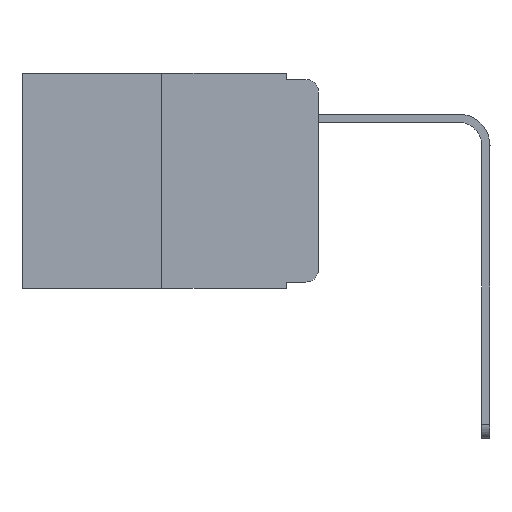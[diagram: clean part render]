
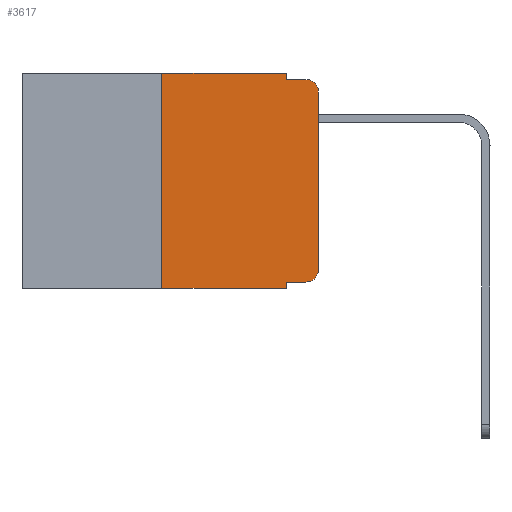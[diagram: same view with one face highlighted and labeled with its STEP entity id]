
A CAD part, left-side view. The second image highlights one B-rep face of the part: STEP entity #3617.
In plain terms, the highlighted planar face has unit normal (-1, 0, 0).
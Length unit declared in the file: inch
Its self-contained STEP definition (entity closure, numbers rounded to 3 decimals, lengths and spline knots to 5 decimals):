
#170 = CARTESIAN_POINT ( 'NONE',  ( 0., 0.02, -0.313 ) ) ;
#175 = VECTOR ( 'NONE', #9931, 39.37008 ) ;
#216 = CARTESIAN_POINT ( 'NONE',  ( 0., 0.02, -0.333 ) ) ;
#273 = LINE ( 'NONE', #3602, #7052 ) ;
#281 = DIRECTION ( 'NONE',  ( 0., 0., -1. ) ) ;
#311 = VERTEX_POINT ( 'NONE', #536 ) ;
#536 = CARTESIAN_POINT ( 'NONE',  ( 0., 0.051, -0.333 ) ) ;
#756 = CARTESIAN_POINT ( 'NONE',  ( 0., 0.051, -0.01 ) ) ;
#774 = CARTESIAN_POINT ( 'NONE',  ( 0., 0.473, -0.343 ) ) ;
#791 = DIRECTION ( 'NONE',  ( 0., 0., -1. ) ) ;
#1147 = VERTEX_POINT ( 'NONE', #8506 ) ;
#1671 = VERTEX_POINT ( 'NONE', #216 ) ;
#1872 = EDGE_CURVE ( 'NONE', #2613, #1147, #7106, .T. ) ;
#2323 = VERTEX_POINT ( 'NONE', #6105 ) ;
#2388 = ORIENTED_EDGE ( 'NONE', *, *, #4063, .T. ) ;
#2407 = LINE ( 'NONE', #8182, #10619 ) ;
#2442 = LINE ( 'NONE', #3770, #7485 ) ;
#2506 = CARTESIAN_POINT ( 'NONE',  ( 0., 0.473, 0. ) ) ;
#2613 = VERTEX_POINT ( 'NONE', #6956 ) ;
#2641 = CIRCLE ( 'NONE', #5296, 0.02 ) ;
#2801 = DIRECTION ( 'NONE',  ( -1., 0., 0. ) ) ;
#2881 = EDGE_CURVE ( 'NONE', #6668, #8296, #2442, .T. ) ;
#2886 = VERTEX_POINT ( 'NONE', #4645 ) ;
#3186 = CARTESIAN_POINT ( 'NONE',  ( 0., 0.051, 0. ) ) ;
#3198 = EDGE_CURVE ( 'NONE', #11571, #2323, #5079, .T. ) ;
#3324 = CARTESIAN_POINT ( 'NONE',  ( 0., 0.25, 0. ) ) ;
#3374 = CARTESIAN_POINT ( 'NONE',  ( 0., 0.25, -0.343 ) ) ;
#3602 = CARTESIAN_POINT ( 'NONE',  ( 0., 0.051, -0.333 ) ) ;
#3617 = ADVANCED_FACE ( 'NONE', ( #4918 ), #4471, .F. ) ;
#3770 = CARTESIAN_POINT ( 'NONE',  ( 0., 0.473, 0. ) ) ;
#3906 = LINE ( 'NONE', #9892, #11394 ) ;
#4063 = EDGE_CURVE ( 'NONE', #2886, #9280, #3906, .T. ) ;
#4388 = ORIENTED_EDGE ( 'NONE', *, *, #8806, .F. ) ;
#4471 = PLANE ( 'NONE',  #6666 ) ;
#4537 = CARTESIAN_POINT ( 'NONE',  ( 0., 0.02, -0.03 ) ) ;
#4572 = CARTESIAN_POINT ( 'NONE',  ( 0., 0.051, 0. ) ) ;
#4645 = CARTESIAN_POINT ( 'NONE',  ( 0., 0., -0.313 ) ) ;
#4918 = FACE_OUTER_BOUND ( 'NONE', #8238, .T. ) ;
#5079 = LINE ( 'NONE', #774, #6542 ) ;
#5296 = AXIS2_PLACEMENT_3D ( 'NONE', #170, #9441, #281 ) ;
#5410 = DIRECTION ( 'NONE',  ( 0., -1., 0. ) ) ;
#5459 = LINE ( 'NONE', #3186, #11064 ) ;
#5646 = DIRECTION ( 'NONE',  ( 0., 0., 1. ) ) ;
#5975 = DIRECTION ( 'NONE',  ( 0., 0., -1. ) ) ;
#6105 = CARTESIAN_POINT ( 'NONE',  ( 0., 0.051, -0.343 ) ) ;
#6279 = AXIS2_PLACEMENT_3D ( 'NONE', #4537, #2801, #10952 ) ;
#6292 = CIRCLE ( 'NONE', #6279, 0.02 ) ;
#6353 = EDGE_CURVE ( 'NONE', #1671, #2886, #2641, .T. ) ;
#6424 = ORIENTED_EDGE ( 'NONE', *, *, #11710, .T. ) ;
#6542 = VECTOR ( 'NONE', #5410, 39.37008 ) ;
#6666 = AXIS2_PLACEMENT_3D ( 'NONE', #2506, #8160, #11783 ) ;
#6668 = VERTEX_POINT ( 'NONE', #3324 ) ;
#6786 = ORIENTED_EDGE ( 'NONE', *, *, #3198, .T. ) ;
#6956 = CARTESIAN_POINT ( 'NONE',  ( 0., 0.051, -0.01 ) ) ;
#7052 = VECTOR ( 'NONE', #11009, 39.37008 ) ;
#7106 = LINE ( 'NONE', #756, #175 ) ;
#7156 = EDGE_CURVE ( 'NONE', #311, #2323, #5459, .T. ) ;
#7397 = ORIENTED_EDGE ( 'NONE', *, *, #7156, .F. ) ;
#7485 = VECTOR ( 'NONE', #11164, 39.37008 ) ;
#7863 = ORIENTED_EDGE ( 'NONE', *, *, #10941, .T. ) ;
#7954 = DIRECTION ( 'NONE',  ( 0., 0., 1. ) ) ;
#8160 = DIRECTION ( 'NONE',  ( 1., 0., 0. ) ) ;
#8182 = CARTESIAN_POINT ( 'NONE',  ( 0., 0.25, 0. ) ) ;
#8238 = EDGE_LOOP ( 'NONE', ( #2388, #6424, #8881, #4388, #8958, #9609, #6786, #7397, #7863, #9768 ) ) ;
#8296 = VERTEX_POINT ( 'NONE', #11800 ) ;
#8461 = EDGE_CURVE ( 'NONE', #11571, #6668, #2407, .T. ) ;
#8506 = CARTESIAN_POINT ( 'NONE',  ( 0., 0.02, -0.01 ) ) ;
#8806 = EDGE_CURVE ( 'NONE', #8296, #2613, #11043, .T. ) ;
#8881 = ORIENTED_EDGE ( 'NONE', *, *, #1872, .F. ) ;
#8958 = ORIENTED_EDGE ( 'NONE', *, *, #2881, .F. ) ;
#9280 = VERTEX_POINT ( 'NONE', #10658 ) ;
#9441 = DIRECTION ( 'NONE',  ( -1., 0., 0. ) ) ;
#9609 = ORIENTED_EDGE ( 'NONE', *, *, #8461, .F. ) ;
#9768 = ORIENTED_EDGE ( 'NONE', *, *, #6353, .T. ) ;
#9892 = CARTESIAN_POINT ( 'NONE',  ( 0., 0., 0. ) ) ;
#9924 = VECTOR ( 'NONE', #791, 39.37008 ) ;
#9931 = DIRECTION ( 'NONE',  ( 0., -1., 0. ) ) ;
#10619 = VECTOR ( 'NONE', #5646, 39.37008 ) ;
#10658 = CARTESIAN_POINT ( 'NONE',  ( 0., 0., -0.03 ) ) ;
#10941 = EDGE_CURVE ( 'NONE', #311, #1671, #273, .T. ) ;
#10952 = DIRECTION ( 'NONE',  ( 0., 0., -1. ) ) ;
#11009 = DIRECTION ( 'NONE',  ( 0., -1., 0. ) ) ;
#11043 = LINE ( 'NONE', #4572, #9924 ) ;
#11064 = VECTOR ( 'NONE', #5975, 39.37008 ) ;
#11164 = DIRECTION ( 'NONE',  ( 0., -1., 0. ) ) ;
#11394 = VECTOR ( 'NONE', #7954, 39.37008 ) ;
#11571 = VERTEX_POINT ( 'NONE', #3374 ) ;
#11710 = EDGE_CURVE ( 'NONE', #9280, #1147, #6292, .T. ) ;
#11783 = DIRECTION ( 'NONE',  ( 0., 0., -1. ) ) ;
#11800 = CARTESIAN_POINT ( 'NONE',  ( 0., 0.051, 0. ) ) ;
